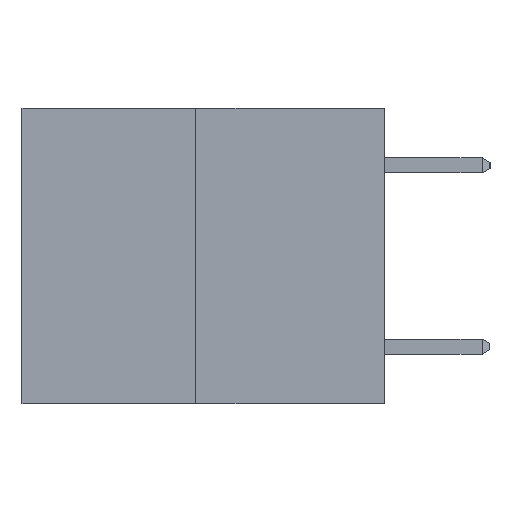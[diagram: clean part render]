
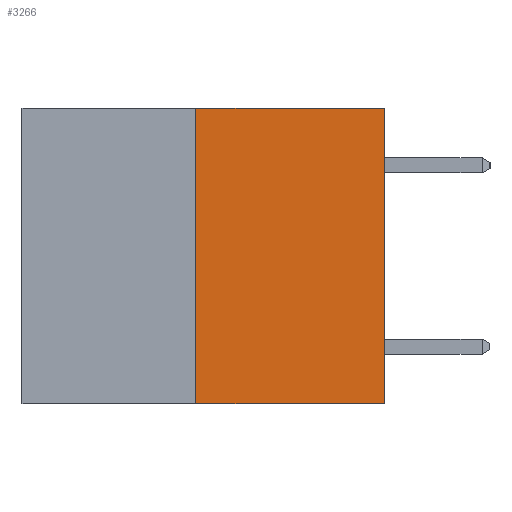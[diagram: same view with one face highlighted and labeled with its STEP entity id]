
A CAD part, left-side view. The second image highlights one B-rep face of the part: STEP entity #3266.
In plain terms, the highlighted planar face has unit normal (-1, 0, 0).
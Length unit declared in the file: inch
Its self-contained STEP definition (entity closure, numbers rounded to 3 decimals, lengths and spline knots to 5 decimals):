
#120 = DIRECTION ( 'NONE',  ( 0., -1., 0. ) ) ;
#238 = CARTESIAN_POINT ( 'NONE',  ( 0., 0.6, -0.49 ) ) ;
#690 = EDGE_CURVE ( 'NONE', #7127, #3879, #9018, .T. ) ;
#817 = CARTESIAN_POINT ( 'NONE',  ( 0., 0.312, -0.49 ) ) ;
#879 = VERTEX_POINT ( 'NONE', #6895 ) ;
#910 = CARTESIAN_POINT ( 'NONE',  ( 0., 0.6, 0. ) ) ;
#1645 = EDGE_CURVE ( 'NONE', #7127, #879, #4623, .T. ) ;
#1786 = VECTOR ( 'NONE', #6006, 39.37008 ) ;
#2612 = PLANE ( 'NONE',  #7961 ) ;
#2641 = ORIENTED_EDGE ( 'NONE', *, *, #5408, .T. ) ;
#3266 = ADVANCED_FACE ( 'NONE', ( #5395 ), #2612, .F. ) ;
#3840 = CARTESIAN_POINT ( 'NONE',  ( 0., 0., 0. ) ) ;
#3879 = VERTEX_POINT ( 'NONE', #5991 ) ;
#4623 = LINE ( 'NONE', #7196, #9285 ) ;
#5247 = ORIENTED_EDGE ( 'NONE', *, *, #690, .T. ) ;
#5318 = EDGE_LOOP ( 'NONE', ( #6770, #5247, #2641, #10491 ) ) ;
#5395 = FACE_OUTER_BOUND ( 'NONE', #5318, .T. ) ;
#5408 = EDGE_CURVE ( 'NONE', #3879, #8213, #11101, .T. ) ;
#5853 = CARTESIAN_POINT ( 'NONE',  ( 0., 0., 0. ) ) ;
#5932 = DIRECTION ( 'NONE',  ( 1., 0., 0. ) ) ;
#5991 = CARTESIAN_POINT ( 'NONE',  ( 0., 0., -0.49 ) ) ;
#6006 = DIRECTION ( 'NONE',  ( 0., -1., 0. ) ) ;
#6431 = DIRECTION ( 'NONE',  ( 0., 0., 1. ) ) ;
#6770 = ORIENTED_EDGE ( 'NONE', *, *, #1645, .F. ) ;
#6895 = CARTESIAN_POINT ( 'NONE',  ( 0., 0.312, 0. ) ) ;
#6936 = DIRECTION ( 'NONE',  ( 0., 0., -1. ) ) ;
#7127 = VERTEX_POINT ( 'NONE', #817 ) ;
#7196 = CARTESIAN_POINT ( 'NONE',  ( 0., 0.312, -0.49 ) ) ;
#7404 = VECTOR ( 'NONE', #8972, 39.37008 ) ;
#7465 = LINE ( 'NONE', #910, #9255 ) ;
#7849 = CARTESIAN_POINT ( 'NONE',  ( 0., 0.6, 0. ) ) ;
#7961 = AXIS2_PLACEMENT_3D ( 'NONE', #7849, #5932, #6936 ) ;
#8213 = VERTEX_POINT ( 'NONE', #5853 ) ;
#8972 = DIRECTION ( 'NONE',  ( 0., 0., 1. ) ) ;
#9018 = LINE ( 'NONE', #238, #1786 ) ;
#9255 = VECTOR ( 'NONE', #120, 39.37008 ) ;
#9285 = VECTOR ( 'NONE', #6431, 39.37008 ) ;
#9650 = EDGE_CURVE ( 'NONE', #879, #8213, #7465, .T. ) ;
#10491 = ORIENTED_EDGE ( 'NONE', *, *, #9650, .F. ) ;
#11101 = LINE ( 'NONE', #3840, #7404 ) ;
